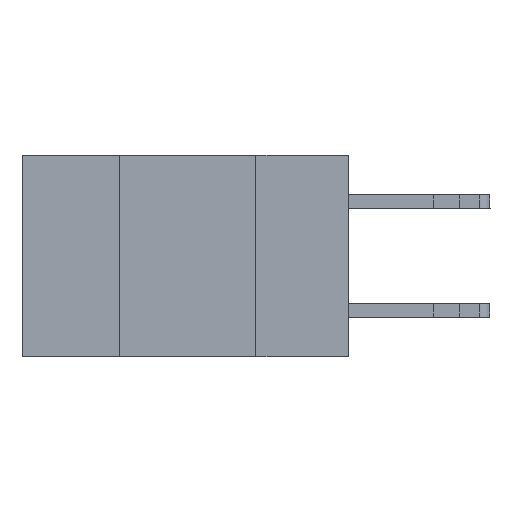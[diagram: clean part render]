
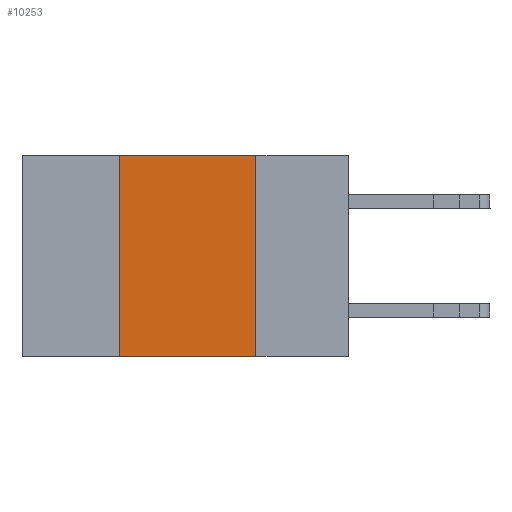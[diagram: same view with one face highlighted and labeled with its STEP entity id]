
A CAD part, left-side view. The second image highlights one B-rep face of the part: STEP entity #10253.
In plain terms, the highlighted planar face has unit normal (-1, 0, 0).
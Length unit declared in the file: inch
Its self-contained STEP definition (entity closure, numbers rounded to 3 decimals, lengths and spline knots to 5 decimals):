
#342 = DIRECTION ( 'NONE',  ( 0., 0., 1. ) ) ;
#521 = EDGE_CURVE ( 'NONE', #8484, #5808, #9236, .T. ) ;
#553 = ORIENTED_EDGE ( 'NONE', *, *, #10544, .T. ) ;
#604 = EDGE_CURVE ( 'NONE', #9925, #8484, #6149, .T. ) ;
#822 = DIRECTION ( 'NONE',  ( 0., 0., -1. ) ) ;
#908 = FACE_OUTER_BOUND ( 'NONE', #12717, .T. ) ;
#976 = DIRECTION ( 'NONE',  ( 1., 0., 0. ) ) ;
#1141 = VECTOR ( 'NONE', #6301, 39.37008 ) ;
#1696 = CARTESIAN_POINT ( 'NONE',  ( 0., 0.6, -0.37 ) ) ;
#1860 = AXIS2_PLACEMENT_3D ( 'NONE', #11071, #976, #12211 ) ;
#3649 = EDGE_CURVE ( 'NONE', #5808, #13684, #6565, .T. ) ;
#3969 = CARTESIAN_POINT ( 'NONE',  ( 0., 0.42, -0.37 ) ) ;
#4648 = DIRECTION ( 'NONE',  ( 0., -1., 0. ) ) ;
#4800 = CARTESIAN_POINT ( 'NONE',  ( 0., 0.6, 0. ) ) ;
#4825 = VECTOR ( 'NONE', #342, 39.37008 ) ;
#5048 = ORIENTED_EDGE ( 'NONE', *, *, #521, .F. ) ;
#5438 = PLANE ( 'NONE',  #1860 ) ;
#5808 = VERTEX_POINT ( 'NONE', #11890 ) ;
#6149 = LINE ( 'NONE', #13039, #4825 ) ;
#6301 = DIRECTION ( 'NONE',  ( 0., -1., 0. ) ) ;
#6453 = ORIENTED_EDGE ( 'NONE', *, *, #3649, .F. ) ;
#6565 = LINE ( 'NONE', #11135, #7580 ) ;
#7013 = VECTOR ( 'NONE', #4648, 39.37008 ) ;
#7580 = VECTOR ( 'NONE', #822, 39.37008 ) ;
#8484 = VERTEX_POINT ( 'NONE', #12232 ) ;
#8950 = LINE ( 'NONE', #1696, #1141 ) ;
#9236 = LINE ( 'NONE', #4800, #7013 ) ;
#9526 = CARTESIAN_POINT ( 'NONE',  ( 0., 0.17, -0.37 ) ) ;
#9925 = VERTEX_POINT ( 'NONE', #3969 ) ;
#10253 = ADVANCED_FACE ( 'NONE', ( #908 ), #5438, .F. ) ;
#10544 = EDGE_CURVE ( 'NONE', #9925, #13684, #8950, .T. ) ;
#11071 = CARTESIAN_POINT ( 'NONE',  ( 0., 0.6, 0. ) ) ;
#11135 = CARTESIAN_POINT ( 'NONE',  ( 0., 0.17, -0.37 ) ) ;
#11890 = CARTESIAN_POINT ( 'NONE',  ( 0., 0.17, 0. ) ) ;
#12211 = DIRECTION ( 'NONE',  ( 0., 0., -1. ) ) ;
#12232 = CARTESIAN_POINT ( 'NONE',  ( 0., 0.42, 0. ) ) ;
#12717 = EDGE_LOOP ( 'NONE', ( #6453, #5048, #12789, #553 ) ) ;
#12789 = ORIENTED_EDGE ( 'NONE', *, *, #604, .F. ) ;
#13039 = CARTESIAN_POINT ( 'NONE',  ( 0., 0.42, -0.37 ) ) ;
#13684 = VERTEX_POINT ( 'NONE', #9526 ) ;
